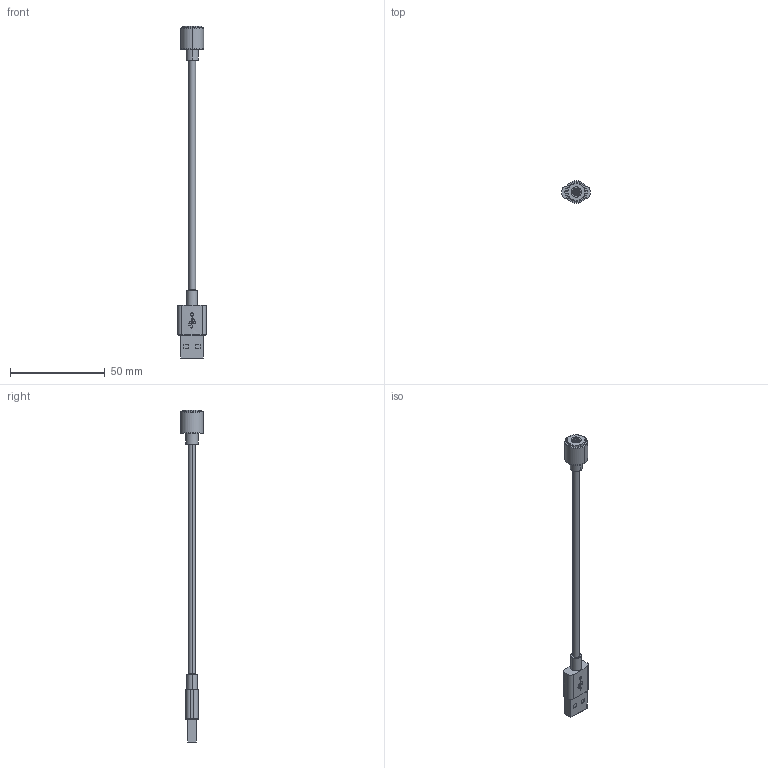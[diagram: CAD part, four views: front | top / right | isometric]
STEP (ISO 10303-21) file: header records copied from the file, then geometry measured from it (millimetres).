
FILE_DESCRIPTION (( 'STEP AP214' ), '1' );
FILE_NAME ('687D0231A000D00.STEP', '2023-04-27T19:21:26', ( '' ), ( '' ), 'SwSTEP 2.0', 'SolidWorks 2020', '' );
FILE_SCHEMA (( 'AUTOMOTIVE_DESIGN' ));
Length unit declared in the file: millimetre
Products named in the file (1): 687D0231A000D00
Bounding box: 14.8 x 12 x 174.79 mm (x, y, z)
Surface area: 4206 mm2 (no closed solid volume)
Topology: 0 solids, 7 shells, 156 faces, 386 edges, 253 vertices
Faces by surface type: plane 71, cylinder 49, torus 18, bspline 10, sphere 4, cone 4
Entity records: 6003 total; most frequent: CARTESIAN_POINT 1427, ORIENTED_EDGE 760, DIRECTION 721, EDGE_CURVE 382, AXIS2_PLACEMENT_3D 273, VERTEX_POINT 253, EDGE_LOOP 181, VECTOR 175
